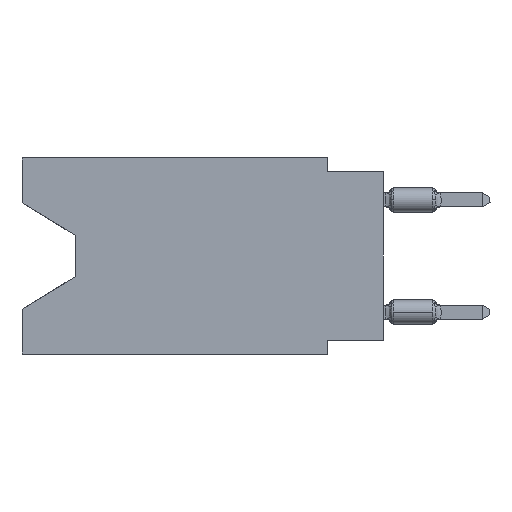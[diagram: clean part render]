
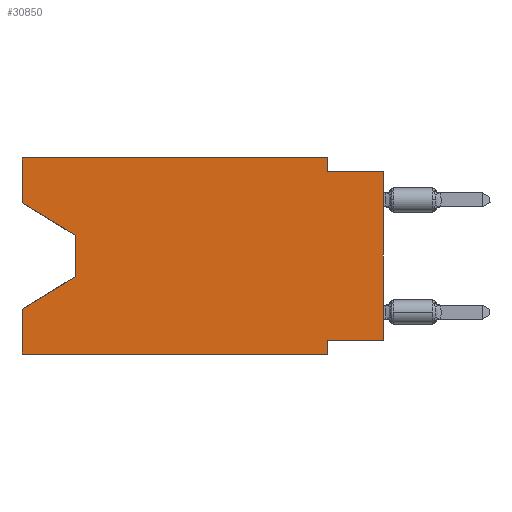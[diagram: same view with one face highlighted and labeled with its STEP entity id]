
A CAD part, left-side view. The second image highlights one B-rep face of the part: STEP entity #30850.
In plain terms, the highlighted planar face has unit normal (-1, 0, 0).
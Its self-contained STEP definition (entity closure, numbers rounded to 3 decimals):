
#59 = DIRECTION ( 'NONE',  ( 0., 0., 1. ) ) ;
#72 = LINE ( 'NONE', #59470, #41261 ) ;
#101 = EDGE_LOOP ( 'NONE', ( #55484, #7505, #58475, #63649, #58765, #14890, #6676, #47318, #62809, #44873, #335, #27017 ) ) ;
#335 = ORIENTED_EDGE ( 'NONE', *, *, #55872, .F. ) ;
#366 = CARTESIAN_POINT ( 'NONE',  ( 0., 16.383, 0. ) ) ;
#529 = CARTESIAN_POINT ( 'NONE',  ( 0., 16.383, 0. ) ) ;
#724 = LINE ( 'NONE', #20856, #14206 ) ;
#1352 = VERTEX_POINT ( 'NONE', #16999 ) ;
#2283 = LINE ( 'NONE', #7780, #42529 ) ;
#2302 = DIRECTION ( 'NONE',  ( 0., -1., 0. ) ) ;
#2599 = VERTEX_POINT ( 'NONE', #9513 ) ;
#4848 = CARTESIAN_POINT ( 'NONE',  ( 0., 16.383, 0. ) ) ;
#5163 = EDGE_CURVE ( 'NONE', #23811, #1352, #72, .T. ) ;
#5180 = FACE_OUTER_BOUND ( 'NONE', #101, .T. ) ;
#6603 = EDGE_CURVE ( 'NONE', #38956, #23313, #32494, .T. ) ;
#6676 = ORIENTED_EDGE ( 'NONE', *, *, #10906, .F. ) ;
#6723 = CARTESIAN_POINT ( 'NONE',  ( 0., 2.54, -8.255 ) ) ;
#7505 = ORIENTED_EDGE ( 'NONE', *, *, #53012, .T. ) ;
#7780 = CARTESIAN_POINT ( 'NONE',  ( 0., 16.383, -2.038 ) ) ;
#9513 = CARTESIAN_POINT ( 'NONE',  ( 0., 2.54, -0.635 ) ) ;
#9731 = CARTESIAN_POINT ( 'NONE',  ( 0., 0., -8.255 ) ) ;
#10319 = DIRECTION ( 'NONE',  ( 0., 0.855, -0.519 ) ) ;
#10906 = EDGE_CURVE ( 'NONE', #23811, #60248, #54672, .T. ) ;
#11125 = CARTESIAN_POINT ( 'NONE',  ( 0., 2.54, 0. ) ) ;
#13914 = DIRECTION ( 'NONE',  ( 0., 0., -1. ) ) ;
#14206 = VECTOR ( 'NONE', #20526, 1000. ) ;
#14890 = ORIENTED_EDGE ( 'NONE', *, *, #63408, .F. ) ;
#14991 = DIRECTION ( 'NONE',  ( 0., 0., 1. ) ) ;
#16113 = CARTESIAN_POINT ( 'NONE',  ( 0., 16.383, -8.89 ) ) ;
#16286 = EDGE_CURVE ( 'NONE', #45959, #58402, #59781, .T. ) ;
#16999 = CARTESIAN_POINT ( 'NONE',  ( 0., 0., -0.635 ) ) ;
#17969 = EDGE_CURVE ( 'NONE', #27295, #2599, #18810, .T. ) ;
#18810 = LINE ( 'NONE', #38586, #27890 ) ;
#19765 = EDGE_CURVE ( 'NONE', #45959, #23102, #2283, .T. ) ;
#20331 = DIRECTION ( 'NONE',  ( 0., 0., 1. ) ) ;
#20526 = DIRECTION ( 'NONE',  ( 0., 0., -1. ) ) ;
#20856 = CARTESIAN_POINT ( 'NONE',  ( 0., 2.54, -8.89 ) ) ;
#21296 = LINE ( 'NONE', #529, #36370 ) ;
#21997 = VERTEX_POINT ( 'NONE', #62236 ) ;
#22247 = CARTESIAN_POINT ( 'NONE',  ( 0., 16.383, -2.038 ) ) ;
#23102 = VERTEX_POINT ( 'NONE', #46522 ) ;
#23313 = VERTEX_POINT ( 'NONE', #28624 ) ;
#23811 = VERTEX_POINT ( 'NONE', #9731 ) ;
#25510 = LINE ( 'NONE', #49549, #44289 ) ;
#27017 = ORIENTED_EDGE ( 'NONE', *, *, #16286, .F. ) ;
#27295 = VERTEX_POINT ( 'NONE', #11125 ) ;
#27890 = VECTOR ( 'NONE', #13914, 1000. ) ;
#28624 = CARTESIAN_POINT ( 'NONE',  ( 0., 2.54, -8.89 ) ) ;
#28833 = VECTOR ( 'NONE', #48059, 1000. ) ;
#30850 = ADVANCED_FACE ( 'NONE', ( #5180 ), #44770, .F. ) ;
#31171 = DIRECTION ( 'NONE',  ( 0., -0.855, -0.519 ) ) ;
#31463 = EDGE_CURVE ( 'NONE', #38956, #21997, #21296, .T. ) ;
#32494 = LINE ( 'NONE', #52300, #28833 ) ;
#34004 = VECTOR ( 'NONE', #44493, 1000. ) ;
#34385 = DIRECTION ( 'NONE',  ( 0., 0., -1. ) ) ;
#34840 = DIRECTION ( 'NONE',  ( 0., 1., 0. ) ) ;
#35234 = AXIS2_PLACEMENT_3D ( 'NONE', #4848, #38907, #34385 ) ;
#36181 = EDGE_CURVE ( 'NONE', #58641, #21997, #45692, .T. ) ;
#36370 = VECTOR ( 'NONE', #20331, 1000. ) ;
#38586 = CARTESIAN_POINT ( 'NONE',  ( 0., 2.54, 0. ) ) ;
#38907 = DIRECTION ( 'NONE',  ( 1., 0., 0. ) ) ;
#38956 = VERTEX_POINT ( 'NONE', #16113 ) ;
#39621 = CARTESIAN_POINT ( 'NONE',  ( 0., 13.97, -3.505 ) ) ;
#40709 = VECTOR ( 'NONE', #34840, 1000. ) ;
#41261 = VECTOR ( 'NONE', #14991, 1000. ) ;
#42148 = CARTESIAN_POINT ( 'NONE',  ( 0., 16.383, 0. ) ) ;
#42529 = VECTOR ( 'NONE', #31171, 1000. ) ;
#44289 = VECTOR ( 'NONE', #54751, 1000. ) ;
#44493 = DIRECTION ( 'NONE',  ( 0., 0., -1. ) ) ;
#44770 = PLANE ( 'NONE',  #35234 ) ;
#44873 = ORIENTED_EDGE ( 'NONE', *, *, #17969, .F. ) ;
#45692 = LINE ( 'NONE', #54799, #63659 ) ;
#45758 = CARTESIAN_POINT ( 'NONE',  ( 0., 13.97, -5.385 ) ) ;
#45959 = VERTEX_POINT ( 'NONE', #22247 ) ;
#46522 = CARTESIAN_POINT ( 'NONE',  ( 0., 13.97, -3.505 ) ) ;
#46760 = CARTESIAN_POINT ( 'NONE',  ( 0., 16.383, 0. ) ) ;
#47318 = ORIENTED_EDGE ( 'NONE', *, *, #5163, .T. ) ;
#48059 = DIRECTION ( 'NONE',  ( 0., -1., 0. ) ) ;
#49049 = LINE ( 'NONE', #39621, #34004 ) ;
#49549 = CARTESIAN_POINT ( 'NONE',  ( 0., 0., -0.635 ) ) ;
#50071 = EDGE_CURVE ( 'NONE', #2599, #1352, #25510, .T. ) ;
#52300 = CARTESIAN_POINT ( 'NONE',  ( 0., 16.383, -8.89 ) ) ;
#53012 = EDGE_CURVE ( 'NONE', #23102, #58641, #49049, .T. ) ;
#54499 = VECTOR ( 'NONE', #2302, 1000. ) ;
#54672 = LINE ( 'NONE', #59531, #40709 ) ;
#54675 = VECTOR ( 'NONE', #59, 1000. ) ;
#54751 = DIRECTION ( 'NONE',  ( 0., -1., 0. ) ) ;
#54799 = CARTESIAN_POINT ( 'NONE',  ( 0., 13.97, -5.385 ) ) ;
#55484 = ORIENTED_EDGE ( 'NONE', *, *, #19765, .T. ) ;
#55872 = EDGE_CURVE ( 'NONE', #58402, #27295, #56843, .T. ) ;
#56843 = LINE ( 'NONE', #46760, #54499 ) ;
#58402 = VERTEX_POINT ( 'NONE', #42148 ) ;
#58475 = ORIENTED_EDGE ( 'NONE', *, *, #36181, .T. ) ;
#58641 = VERTEX_POINT ( 'NONE', #45758 ) ;
#58765 = ORIENTED_EDGE ( 'NONE', *, *, #6603, .T. ) ;
#59470 = CARTESIAN_POINT ( 'NONE',  ( 0., 0., 0. ) ) ;
#59531 = CARTESIAN_POINT ( 'NONE',  ( 0., 0., -8.255 ) ) ;
#59781 = LINE ( 'NONE', #366, #54675 ) ;
#60248 = VERTEX_POINT ( 'NONE', #6723 ) ;
#62236 = CARTESIAN_POINT ( 'NONE',  ( 0., 16.383, -6.852 ) ) ;
#62809 = ORIENTED_EDGE ( 'NONE', *, *, #50071, .F. ) ;
#63408 = EDGE_CURVE ( 'NONE', #60248, #23313, #724, .T. ) ;
#63649 = ORIENTED_EDGE ( 'NONE', *, *, #31463, .F. ) ;
#63659 = VECTOR ( 'NONE', #10319, 1000. ) ;
